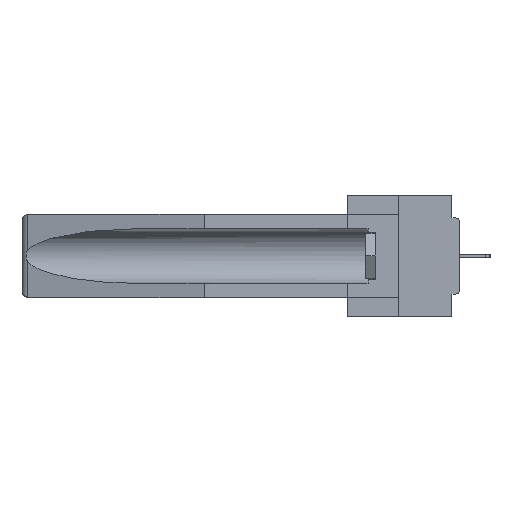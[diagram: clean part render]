
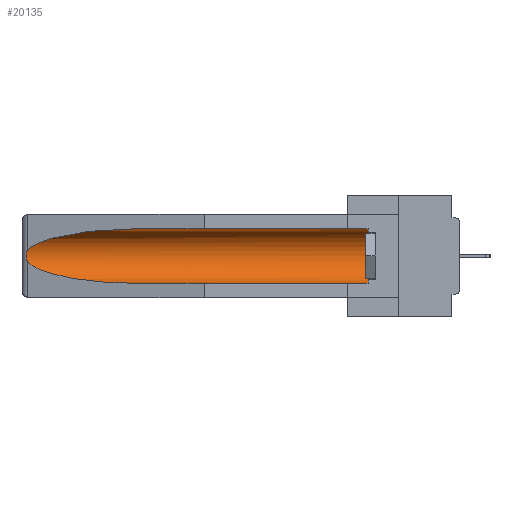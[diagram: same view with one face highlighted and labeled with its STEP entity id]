
A CAD part, left-side view. The second image highlights one B-rep face of the part: STEP entity #20135.
In plain terms, the highlighted cylindrical face has radius 2.857 mm (diameter 5.715 mm), a partial arc.
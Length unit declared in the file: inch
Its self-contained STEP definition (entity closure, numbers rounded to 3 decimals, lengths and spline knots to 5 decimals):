
#329 = CARTESIAN_POINT ( 'NONE',  ( 0.26537, 1.52718, -0.19328 ) ) ;
#330 = ORIENTED_EDGE ( 'NONE', *, *, #18851, .T. ) ;
#488 = CARTESIAN_POINT ( 'NONE',  ( 0.155, -0.30754, -0.059 ) ) ;
#1065 = VERTEX_POINT ( 'NONE', #17443 ) ;
#1434 = DIRECTION ( 'NONE',  ( 0., 0., 1. ) ) ;
#2971 = CARTESIAN_POINT ( 'NONE',  ( 0.21114, 1.30732, -0.059 ) ) ;
#3010 = CARTESIAN_POINT ( 'NONE',  ( 0.26597, 1.5296, -0.19026 ) ) ;
#3353 = ORIENTED_EDGE ( 'NONE', *, *, #9346, .T. ) ;
#3539 = CARTESIAN_POINT ( 'NONE',  ( 0.155, -0.30754, -0.284 ) ) ;
#3645 = CARTESIAN_POINT ( 'NONE',  ( 0.155, 1.07973, -0.284 ) ) ;
#4020 =( BOUNDED_CURVE ( )  B_SPLINE_CURVE ( 3, ( #5854, #25084, #22706, #3645 ),
 .UNSPECIFIED., .F., .T. ) 
 B_SPLINE_CURVE_WITH_KNOTS ( ( 4, 4 ),
 ( 0.1948, 1.5708 ),
 .UNSPECIFIED. ) 
 CURVE ( )  GEOMETRIC_REPRESENTATION_ITEM ( )  RATIONAL_B_SPLINE_CURVE ( ( 1., 0.848, 0.848, 1. ) ) 
 REPRESENTATION_ITEM ( '' )  );
#4309 = VERTEX_POINT ( 'NONE', #20867 ) ;
#4743 = CARTESIAN_POINT ( 'NONE',  ( 0.26597, 1.52961, -0.15275 ) ) ;
#5214 = DIRECTION ( 'NONE',  ( 0., 0., 1. ) ) ;
#5702 = B_SPLINE_CURVE_WITH_KNOTS ( 'NONE', 3,
 ( #26336, #4743, #23965, #12626, #7848, #19389, #24134, #14679, #3010, #329 ),
 .UNSPECIFIED., .F., .F.,
 ( 4, 2, 2, 2, 4 ),
 ( 0., 0.00029, 0.00058, 0.00087, 0.00117 ),
 .UNSPECIFIED. ) ;
#5854 = CARTESIAN_POINT ( 'NONE',  ( 0.26537, 1.52718, -0.19328 ) ) ;
#5858 = AXIS2_PLACEMENT_3D ( 'NONE', #5981, #8331, #1434 ) ;
#5981 = CARTESIAN_POINT ( 'NONE',  ( 0.155, 0.126, -0.1715 ) ) ;
#6403 = CARTESIAN_POINT ( 'NONE',  ( 0.155, 1.07973, -0.059 ) ) ;
#7848 = CARTESIAN_POINT ( 'NONE',  ( 0.2675, 1.53308, -0.16763 ) ) ;
#7865 = CYLINDRICAL_SURFACE ( 'NONE', #29663, 0.1125 ) ;
#8331 = DIRECTION ( 'NONE',  ( 0., -1., 0. ) ) ;
#8346 = ORIENTED_EDGE ( 'NONE', *, *, #24264, .T. ) ;
#8391 = LINE ( 'NONE', #3539, #11677 ) ;
#8855 = VERTEX_POINT ( 'NONE', #31145 ) ;
#9084 = EDGE_CURVE ( 'NONE', #4309, #8855, #8391, .T. ) ;
#9346 = EDGE_CURVE ( 'NONE', #18429, #30665, #12456, .T. ) ;
#9936 = DIRECTION ( 'NONE',  ( 0., 1., 0. ) ) ;
#10535 = CARTESIAN_POINT ( 'NONE',  ( 0.155, 1.07973, -0.059 ) ) ;
#11208 = VECTOR ( 'NONE', #9936, 39.37008 ) ;
#11677 = VECTOR ( 'NONE', #24811, 39.37008 ) ;
#11836 = CARTESIAN_POINT ( 'NONE',  ( 0.26537, 1.52718, -0.19328 ) ) ;
#12456 = LINE ( 'NONE', #488, #11208 ) ;
#12626 = CARTESIAN_POINT ( 'NONE',  ( 0.2673, 1.5327, -0.16383 ) ) ;
#12640 = CARTESIAN_POINT ( 'NONE',  ( 0.155, -0.30754, -0.1715 ) ) ;
#12734 = CARTESIAN_POINT ( 'NONE',  ( 0.25451, 1.48313, -0.09465 ) ) ;
#12846 = VERTEX_POINT ( 'NONE', #11836 ) ;
#14679 = CARTESIAN_POINT ( 'NONE',  ( 0.26655, 1.53094, -0.18657 ) ) ;
#14847 = DIRECTION ( 'NONE',  ( 0., 1., 0. ) ) ;
#15416 = CARTESIAN_POINT ( 'NONE',  ( 0.26537, 1.52718, -0.14972 ) ) ;
#15901 =( BOUNDED_CURVE ( )  B_SPLINE_CURVE ( 3, ( #10535, #2971, #12734, #15416 ),
 .UNSPECIFIED., .F., .F. ) 
 B_SPLINE_CURVE_WITH_KNOTS ( ( 4, 4 ),
 ( 4.71239, 6.08839 ),
 .UNSPECIFIED. ) 
 CURVE ( )  GEOMETRIC_REPRESENTATION_ITEM ( )  RATIONAL_B_SPLINE_CURVE ( ( 1., 0.848, 0.848, 1. ) ) 
 REPRESENTATION_ITEM ( '' )  );
#17443 = CARTESIAN_POINT ( 'NONE',  ( 0.26537, 1.52718, -0.14972 ) ) ;
#17732 = EDGE_CURVE ( 'NONE', #12846, #8855, #4020, .T. ) ;
#18372 = ORIENTED_EDGE ( 'NONE', *, *, #9084, .F. ) ;
#18429 = VERTEX_POINT ( 'NONE', #26367 ) ;
#18851 = EDGE_CURVE ( 'NONE', #1065, #12846, #5702, .T. ) ;
#19389 = CARTESIAN_POINT ( 'NONE',  ( 0.2675, 1.53308, -0.17534 ) ) ;
#20028 = FACE_OUTER_BOUND ( 'NONE', #24982, .T. ) ;
#20135 = ADVANCED_FACE ( 'NONE', ( #20028 ), #7865, .F. ) ;
#20867 = CARTESIAN_POINT ( 'NONE',  ( 0.155, 0.126, -0.284 ) ) ;
#22359 = ORIENTED_EDGE ( 'NONE', *, *, #26328, .T. ) ;
#22706 = CARTESIAN_POINT ( 'NONE',  ( 0.21114, 1.30732, -0.284 ) ) ;
#23965 = CARTESIAN_POINT ( 'NONE',  ( 0.26654, 1.53092, -0.15636 ) ) ;
#24134 = CARTESIAN_POINT ( 'NONE',  ( 0.2673, 1.53269, -0.17917 ) ) ;
#24264 = EDGE_CURVE ( 'NONE', #30665, #1065, #15901, .T. ) ;
#24811 = DIRECTION ( 'NONE',  ( 0., 1., 0. ) ) ;
#24982 = EDGE_LOOP ( 'NONE', ( #8346, #330, #26663, #18372, #22359, #3353 ) ) ;
#25084 = CARTESIAN_POINT ( 'NONE',  ( 0.25451, 1.48313, -0.24835 ) ) ;
#26328 = EDGE_CURVE ( 'NONE', #4309, #18429, #31051, .T. ) ;
#26336 = CARTESIAN_POINT ( 'NONE',  ( 0.26537, 1.52718, -0.14972 ) ) ;
#26367 = CARTESIAN_POINT ( 'NONE',  ( 0.155, 0.126, -0.059 ) ) ;
#26663 = ORIENTED_EDGE ( 'NONE', *, *, #17732, .T. ) ;
#29663 = AXIS2_PLACEMENT_3D ( 'NONE', #12640, #14847, #5214 ) ;
#30665 = VERTEX_POINT ( 'NONE', #6403 ) ;
#31051 = CIRCLE ( 'NONE', #5858, 0.1125 ) ;
#31145 = CARTESIAN_POINT ( 'NONE',  ( 0.155, 1.07973, -0.284 ) ) ;
